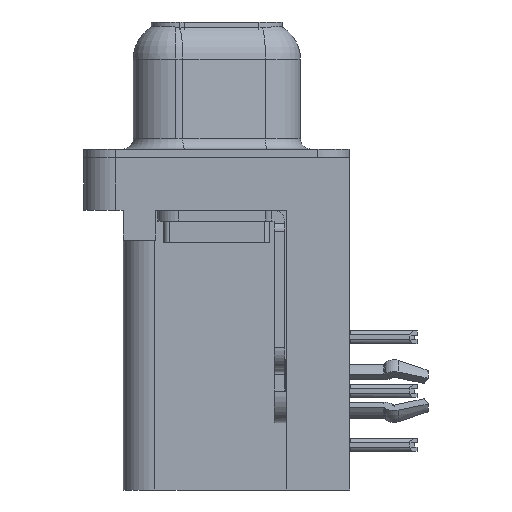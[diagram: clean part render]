
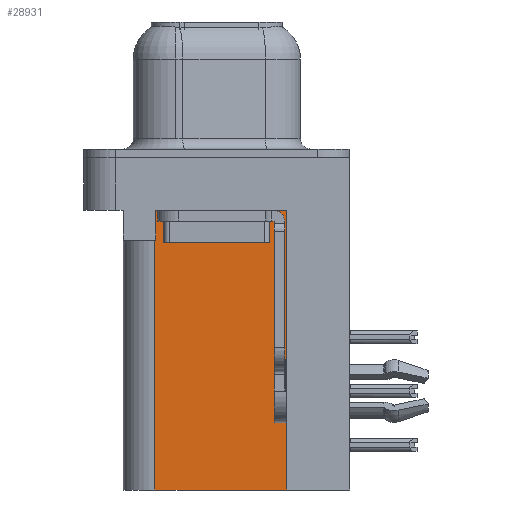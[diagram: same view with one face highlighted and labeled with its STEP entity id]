
A CAD part, left-side view. The second image highlights one B-rep face of the part: STEP entity #28931.
In plain terms, the highlighted planar face has unit normal (-1, 0, 0).
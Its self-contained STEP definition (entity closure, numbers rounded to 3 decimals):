
#74 = CARTESIAN_POINT ( 'NONE',  ( 3.765, 2.925, -15.7 ) ) ;
#2131 = CARTESIAN_POINT ( 'NONE',  ( 3.765, 2.895, -3.9 ) ) ;
#2139 = VECTOR ( 'NONE', #24096, 1000. ) ;
#2271 = LINE ( 'NONE', #30986, #30267 ) ;
#3050 = CARTESIAN_POINT ( 'NONE',  ( 3.765, -3.295, -15.7 ) ) ;
#3240 = VERTEX_POINT ( 'NONE', #34037 ) ;
#3337 = VECTOR ( 'NONE', #17984, 1000. ) ;
#3416 = EDGE_CURVE ( 'NONE', #12159, #21256, #2271, .T. ) ;
#3982 = CARTESIAN_POINT ( 'NONE',  ( 3.765, -3.295, -2.5 ) ) ;
#4541 = DIRECTION ( 'NONE',  ( 0., 1., 0. ) ) ;
#4931 = EDGE_CURVE ( 'NONE', #21256, #11703, #38562, .T. ) ;
#6113 = DIRECTION ( 'NONE',  ( 0., 0., 1. ) ) ;
#6571 = EDGE_CURVE ( 'NONE', #11703, #3240, #19083, .T. ) ;
#7573 = CARTESIAN_POINT ( 'NONE',  ( 3.765, -3.295, -15.7 ) ) ;
#7990 = VECTOR ( 'NONE', #4541, 1000. ) ;
#9180 = DIRECTION ( 'NONE',  ( 0., 1., 0. ) ) ;
#9405 = VECTOR ( 'NONE', #6113, 1000. ) ;
#11549 = EDGE_CURVE ( 'NONE', #19051, #3240, #26362, .T. ) ;
#11703 = VERTEX_POINT ( 'NONE', #33257 ) ;
#12159 = VERTEX_POINT ( 'NONE', #3982 ) ;
#12442 = EDGE_CURVE ( 'NONE', #38428, #19051, #16933, .T. ) ;
#12665 = EDGE_CURVE ( 'NONE', #38428, #12159, #33166, .T. ) ;
#12695 = EDGE_LOOP ( 'NONE', ( #31451, #17139, #35251, #23363, #31226, #25075 ) ) ;
#13399 = CARTESIAN_POINT ( 'NONE',  ( 3.765, -3.295, -15.7 ) ) ;
#16209 = AXIS2_PLACEMENT_3D ( 'NONE', #13399, #34273, #16489 ) ;
#16489 = DIRECTION ( 'NONE',  ( 0., 1., 0. ) ) ;
#16933 = LINE ( 'NONE', #7573, #7990 ) ;
#17139 = ORIENTED_EDGE ( 'NONE', *, *, #4931, .T. ) ;
#17984 = DIRECTION ( 'NONE',  ( 0., 0., 1. ) ) ;
#19051 = VERTEX_POINT ( 'NONE', #36708 ) ;
#19083 = LINE ( 'NONE', #27002, #2139 ) ;
#21256 = VERTEX_POINT ( 'NONE', #35505 ) ;
#23363 = ORIENTED_EDGE ( 'NONE', *, *, #11549, .F. ) ;
#24096 = DIRECTION ( 'NONE',  ( 0., 1., 0. ) ) ;
#25075 = ORIENTED_EDGE ( 'NONE', *, *, #12665, .T. ) ;
#26362 = LINE ( 'NONE', #74, #3337 ) ;
#27002 = CARTESIAN_POINT ( 'NONE',  ( 3.765, 0., -3.9 ) ) ;
#27431 = FACE_OUTER_BOUND ( 'NONE', #12695, .T. ) ;
#28066 = CARTESIAN_POINT ( 'NONE',  ( 3.765, -3.295, -15.7 ) ) ;
#28893 = DIRECTION ( 'NONE',  ( 0., 0., -1. ) ) ;
#28931 = ADVANCED_FACE ( 'NONE', ( #27431 ), #30757, .F. ) ;
#30267 = VECTOR ( 'NONE', #9180, 1000. ) ;
#30757 = PLANE ( 'NONE',  #16209 ) ;
#30986 = CARTESIAN_POINT ( 'NONE',  ( 3.765, -3.295, -2.5 ) ) ;
#31226 = ORIENTED_EDGE ( 'NONE', *, *, #12442, .F. ) ;
#31451 = ORIENTED_EDGE ( 'NONE', *, *, #3416, .T. ) ;
#33166 = LINE ( 'NONE', #3050, #9405 ) ;
#33257 = CARTESIAN_POINT ( 'NONE',  ( 3.765, 2.895, -3.9 ) ) ;
#34037 = CARTESIAN_POINT ( 'NONE',  ( 3.765, 2.925, -3.9 ) ) ;
#34273 = DIRECTION ( 'NONE',  ( 1., 0., 0. ) ) ;
#35251 = ORIENTED_EDGE ( 'NONE', *, *, #6571, .T. ) ;
#35505 = CARTESIAN_POINT ( 'NONE',  ( 3.765, 2.895, -2.5 ) ) ;
#36708 = CARTESIAN_POINT ( 'NONE',  ( 3.765, 2.925, -15.7 ) ) ;
#37658 = VECTOR ( 'NONE', #28893, 1000. ) ;
#38428 = VERTEX_POINT ( 'NONE', #28066 ) ;
#38562 = LINE ( 'NONE', #2131, #37658 ) ;
